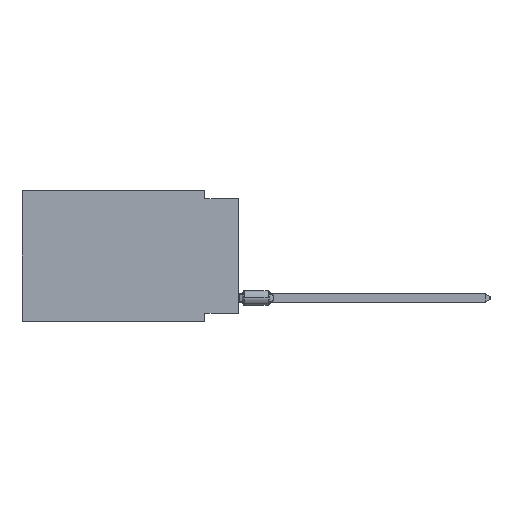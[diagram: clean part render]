
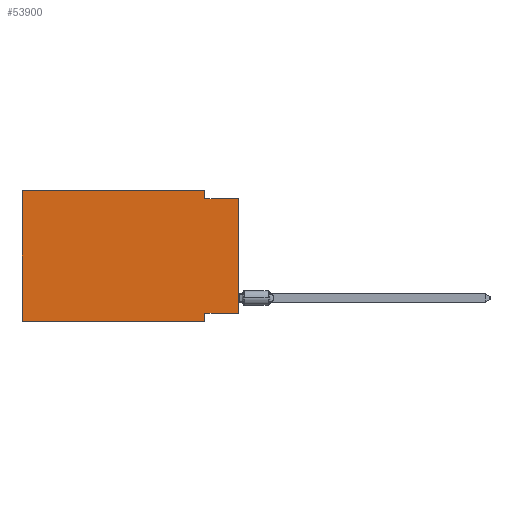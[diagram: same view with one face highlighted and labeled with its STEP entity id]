
A CAD part, left-side view. The second image highlights one B-rep face of the part: STEP entity #53900.
In plain terms, the highlighted planar face has unit normal (-1, 0, 0).
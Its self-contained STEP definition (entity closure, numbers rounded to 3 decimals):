
#2540 = VERTEX_POINT ( 'NONE', #75467 ) ;
#3255 = DIRECTION ( 'NONE',  ( 0., -1., 0. ) ) ;
#5602 = CARTESIAN_POINT ( 'NONE',  ( 0., 2.54, 0. ) ) ;
#5912 = LINE ( 'NONE', #30997, #63393 ) ;
#8505 = EDGE_CURVE ( 'NONE', #9763, #77693, #61219, .T. ) ;
#8801 = CARTESIAN_POINT ( 'NONE',  ( 0., 0., -0.635 ) ) ;
#9763 = VERTEX_POINT ( 'NONE', #75547 ) ;
#10734 = LINE ( 'NONE', #48102, #34153 ) ;
#11244 = ORIENTED_EDGE ( 'NONE', *, *, #39394, .F. ) ;
#12481 = DIRECTION ( 'NONE',  ( 0., 1., 0. ) ) ;
#12762 = VECTOR ( 'NONE', #73530, 1000. ) ;
#13096 = VECTOR ( 'NONE', #3255, 1000. ) ;
#13481 = CARTESIAN_POINT ( 'NONE',  ( 0., 2.54, -9.271 ) ) ;
#14542 = LINE ( 'NONE', #39620, #75076 ) ;
#14807 = VERTEX_POINT ( 'NONE', #8801 ) ;
#15585 = CARTESIAN_POINT ( 'NONE',  ( 0., 0., -0.635 ) ) ;
#16175 = VECTOR ( 'NONE', #54250, 1000. ) ;
#20938 = EDGE_LOOP ( 'NONE', ( #36901, #41988, #11244, #27254, #64753, #31006, #32484, #39426 ) ) ;
#24914 = DIRECTION ( 'NONE',  ( 0., 0., -1. ) ) ;
#25676 = CARTESIAN_POINT ( 'NONE',  ( 0., 2.54, -0.635 ) ) ;
#27254 = ORIENTED_EDGE ( 'NONE', *, *, #70096, .F. ) ;
#30997 = CARTESIAN_POINT ( 'NONE',  ( 0., 0., -9.271 ) ) ;
#31006 = ORIENTED_EDGE ( 'NONE', *, *, #65032, .T. ) ;
#32484 = ORIENTED_EDGE ( 'NONE', *, *, #54895, .F. ) ;
#34153 = VECTOR ( 'NONE', #65805, 1000. ) ;
#34797 = EDGE_CURVE ( 'NONE', #44394, #14807, #10734, .T. ) ;
#34869 = PLANE ( 'NONE',  #59899 ) ;
#36901 = ORIENTED_EDGE ( 'NONE', *, *, #34797, .T. ) ;
#37245 = LINE ( 'NONE', #5602, #55551 ) ;
#38784 = CARTESIAN_POINT ( 'NONE',  ( 0., 0., -9.271 ) ) ;
#39105 = VERTEX_POINT ( 'NONE', #57852 ) ;
#39394 = EDGE_CURVE ( 'NONE', #2540, #66224, #37245, .T. ) ;
#39426 = ORIENTED_EDGE ( 'NONE', *, *, #71211, .F. ) ;
#39620 = CARTESIAN_POINT ( 'NONE',  ( 0., 16.383, 0. ) ) ;
#39841 = DIRECTION ( 'NONE',  ( 0., 0., -1. ) ) ;
#40241 = CARTESIAN_POINT ( 'NONE',  ( 0., 16.383, 0. ) ) ;
#41905 = CARTESIAN_POINT ( 'NONE',  ( 0., 2.54, -9.906 ) ) ;
#41988 = ORIENTED_EDGE ( 'NONE', *, *, #49275, .F. ) ;
#42323 = VERTEX_POINT ( 'NONE', #13481 ) ;
#44394 = VERTEX_POINT ( 'NONE', #38784 ) ;
#45598 = LINE ( 'NONE', #15585, #80603 ) ;
#45988 = FACE_OUTER_BOUND ( 'NONE', #20938, .T. ) ;
#48102 = CARTESIAN_POINT ( 'NONE',  ( 0., 0., 0. ) ) ;
#49275 = EDGE_CURVE ( 'NONE', #66224, #14807, #45598, .T. ) ;
#53396 = LINE ( 'NONE', #41905, #12762 ) ;
#53900 = ADVANCED_FACE ( 'NONE', ( #45988 ), #34869, .F. ) ;
#54250 = DIRECTION ( 'NONE',  ( 0., 0., 1. ) ) ;
#54895 = EDGE_CURVE ( 'NONE', #42323, #39105, #53396, .T. ) ;
#55056 = CARTESIAN_POINT ( 'NONE',  ( 0., 16.383, 0. ) ) ;
#55551 = VECTOR ( 'NONE', #24914, 1000. ) ;
#57852 = CARTESIAN_POINT ( 'NONE',  ( 0., 2.54, -9.906 ) ) ;
#58472 = DIRECTION ( 'NONE',  ( 0., -1., 0. ) ) ;
#58557 = CARTESIAN_POINT ( 'NONE',  ( 0., 16.383, 0. ) ) ;
#59538 = LINE ( 'NONE', #77663, #13096 ) ;
#59899 = AXIS2_PLACEMENT_3D ( 'NONE', #40241, #59901, #39841 ) ;
#59901 = DIRECTION ( 'NONE',  ( 1., 0., 0. ) ) ;
#61219 = LINE ( 'NONE', #55056, #16175 ) ;
#63393 = VECTOR ( 'NONE', #12481, 1000. ) ;
#64753 = ORIENTED_EDGE ( 'NONE', *, *, #8505, .F. ) ;
#64895 = DIRECTION ( 'NONE',  ( 0., -1., 0. ) ) ;
#65032 = EDGE_CURVE ( 'NONE', #9763, #39105, #59538, .T. ) ;
#65805 = DIRECTION ( 'NONE',  ( 0., 0., 1. ) ) ;
#66224 = VERTEX_POINT ( 'NONE', #25676 ) ;
#70096 = EDGE_CURVE ( 'NONE', #77693, #2540, #14542, .T. ) ;
#71211 = EDGE_CURVE ( 'NONE', #44394, #42323, #5912, .T. ) ;
#73530 = DIRECTION ( 'NONE',  ( 0., 0., -1. ) ) ;
#75076 = VECTOR ( 'NONE', #58472, 1000. ) ;
#75467 = CARTESIAN_POINT ( 'NONE',  ( 0., 2.54, 0. ) ) ;
#75547 = CARTESIAN_POINT ( 'NONE',  ( 0., 16.383, -9.906 ) ) ;
#77663 = CARTESIAN_POINT ( 'NONE',  ( 0., 16.383, -9.906 ) ) ;
#77693 = VERTEX_POINT ( 'NONE', #58557 ) ;
#80603 = VECTOR ( 'NONE', #64895, 1000. ) ;
